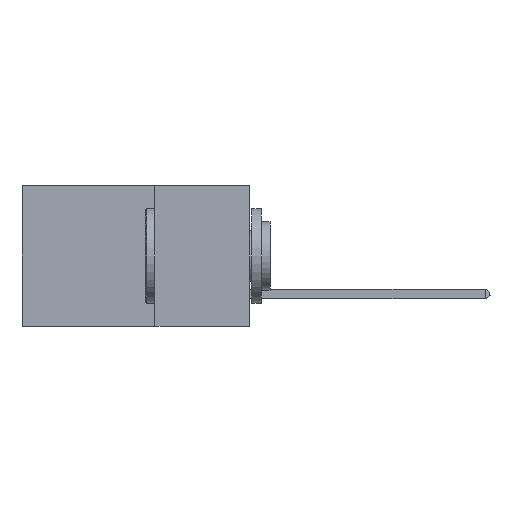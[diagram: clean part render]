
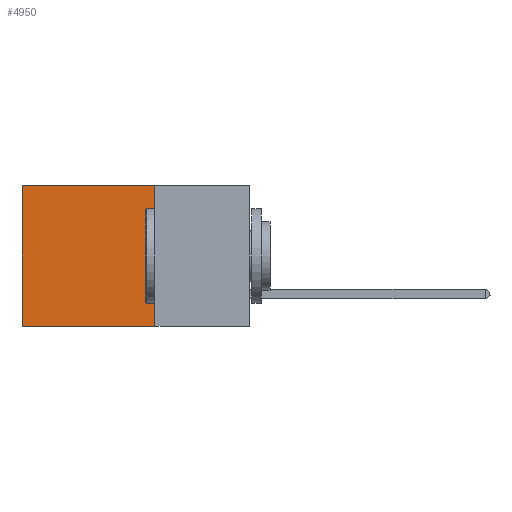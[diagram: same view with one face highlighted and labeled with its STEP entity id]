
A CAD part, left-side view. The second image highlights one B-rep face of the part: STEP entity #4950.
In plain terms, the highlighted planar face has unit normal (-1, 0, 0).
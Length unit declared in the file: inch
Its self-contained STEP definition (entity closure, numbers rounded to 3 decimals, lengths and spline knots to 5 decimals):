
#591 = LINE ( 'NONE', #15907, #13918 ) ;
#852 = CARTESIAN_POINT ( 'NONE',  ( 0.2875, 0.25, 0. ) ) ;
#2685 = ORIENTED_EDGE ( 'NONE', *, *, #23510, .F. ) ;
#2993 = DIRECTION ( 'NONE',  ( 0., 0., -1. ) ) ;
#3383 = PLANE ( 'NONE',  #3634 ) ;
#3634 = AXIS2_PLACEMENT_3D ( 'NONE', #852, #12215, #21631 ) ;
#4513 = ORIENTED_EDGE ( 'NONE', *, *, #14719, .T. ) ;
#4950 = ADVANCED_FACE ( 'NONE', ( #23204 ), #3383, .F. ) ;
#5120 = CARTESIAN_POINT ( 'NONE',  ( 0.2875, 0.25, -0.37 ) ) ;
#5644 = VECTOR ( 'NONE', #6579, 39.37008 ) ;
#6579 = DIRECTION ( 'NONE',  ( 0., 0., -1. ) ) ;
#6842 = EDGE_CURVE ( 'NONE', #12772, #20232, #591, .T. ) ;
#7174 = VERTEX_POINT ( 'NONE', #14083 ) ;
#11019 = LINE ( 'NONE', #21574, #27237 ) ;
#12215 = DIRECTION ( 'NONE',  ( 1., 0., 0. ) ) ;
#12772 = VERTEX_POINT ( 'NONE', #23815 ) ;
#13201 = LINE ( 'NONE', #18578, #5644 ) ;
#13458 = EDGE_LOOP ( 'NONE', ( #4513, #2685, #13867, #28563 ) ) ;
#13867 = ORIENTED_EDGE ( 'NONE', *, *, #14118, .F. ) ;
#13918 = VECTOR ( 'NONE', #18247, 39.37008 ) ;
#14083 = CARTESIAN_POINT ( 'NONE',  ( 0.2875, 0.25, -0.37 ) ) ;
#14118 = EDGE_CURVE ( 'NONE', #12772, #7174, #13201, .T. ) ;
#14648 = CARTESIAN_POINT ( 'NONE',  ( 0.2875, 0.6, 0. ) ) ;
#14719 = EDGE_CURVE ( 'NONE', #20232, #25674, #11019, .T. ) ;
#15907 = CARTESIAN_POINT ( 'NONE',  ( 0.2875, 0.25, 0. ) ) ;
#18247 = DIRECTION ( 'NONE',  ( 0., 1., 0. ) ) ;
#18578 = CARTESIAN_POINT ( 'NONE',  ( 0.2875, 0.25, 0. ) ) ;
#20232 = VERTEX_POINT ( 'NONE', #14648 ) ;
#20814 = LINE ( 'NONE', #5120, #28062 ) ;
#21574 = CARTESIAN_POINT ( 'NONE',  ( 0.2875, 0.6, 0. ) ) ;
#21631 = DIRECTION ( 'NONE',  ( 0., 0., -1. ) ) ;
#23204 = FACE_OUTER_BOUND ( 'NONE', #13458, .T. ) ;
#23510 = EDGE_CURVE ( 'NONE', #7174, #25674, #20814, .T. ) ;
#23621 = DIRECTION ( 'NONE',  ( 0., 1., 0. ) ) ;
#23815 = CARTESIAN_POINT ( 'NONE',  ( 0.2875, 0.25, 0. ) ) ;
#25674 = VERTEX_POINT ( 'NONE', #26883 ) ;
#26883 = CARTESIAN_POINT ( 'NONE',  ( 0.2875, 0.6, -0.37 ) ) ;
#27237 = VECTOR ( 'NONE', #2993, 39.37008 ) ;
#28062 = VECTOR ( 'NONE', #23621, 39.37008 ) ;
#28563 = ORIENTED_EDGE ( 'NONE', *, *, #6842, .T. ) ;
